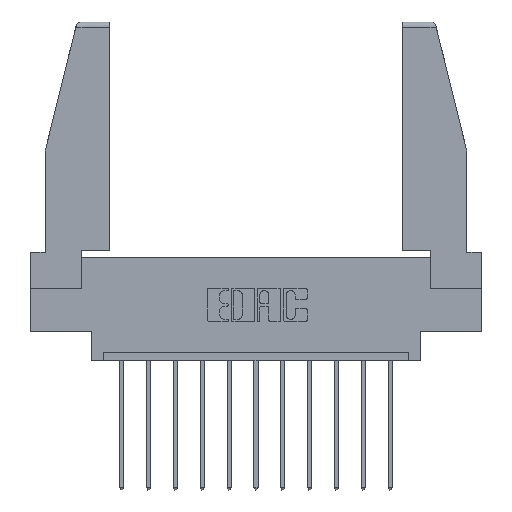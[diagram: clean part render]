
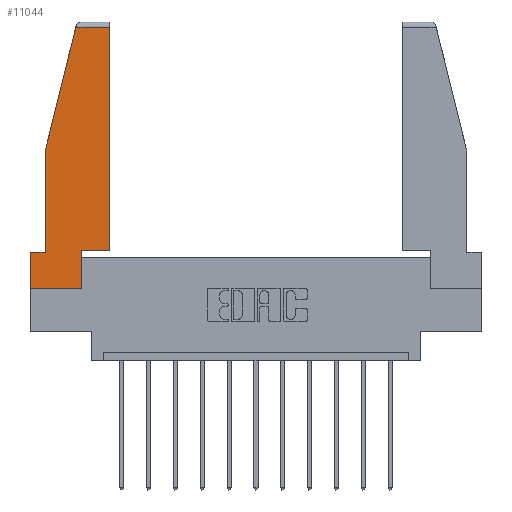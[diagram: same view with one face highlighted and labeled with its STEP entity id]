
A CAD part, top view. The second image highlights one B-rep face of the part: STEP entity #11044.
In plain terms, the highlighted planar face has unit normal (0, 0, 1).
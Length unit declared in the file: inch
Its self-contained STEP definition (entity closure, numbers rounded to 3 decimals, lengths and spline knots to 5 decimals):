
#99 = VERTEX_POINT ( 'NONE', #249 ) ;
#249 = CARTESIAN_POINT ( 'NONE',  ( 0., 0., 0. ) ) ;
#273 = VERTEX_POINT ( 'NONE', #652 ) ;
#368 = DIRECTION ( 'NONE',  ( 1., 0., 0. ) ) ;
#548 = ORIENTED_EDGE ( 'NONE', *, *, #2479, .T. ) ;
#652 = CARTESIAN_POINT ( 'NONE',  ( 0.297, 0., 0. ) ) ;
#979 = VECTOR ( 'NONE', #10877, 39.37008 ) ;
#1027 = CARTESIAN_POINT ( 'NONE',  ( 0.2636, 1.52, 0. ) ) ;
#1032 = PLANE ( 'NONE',  #13003 ) ;
#1252 = VERTEX_POINT ( 'NONE', #6017 ) ;
#1619 = VERTEX_POINT ( 'NONE', #10831 ) ;
#1668 = VERTEX_POINT ( 'NONE', #13361 ) ;
#1780 = EDGE_CURVE ( 'NONE', #8376, #1252, #3135, .T. ) ;
#1925 = VERTEX_POINT ( 'NONE', #1027 ) ;
#1956 = CARTESIAN_POINT ( 'NONE',  ( 0.086, 0.21, 0. ) ) ;
#2058 = EDGE_LOOP ( 'NONE', ( #2463, #4514, #11851, #9837, #10548, #11877, #548, #4662, #4446 ) ) ;
#2217 = CARTESIAN_POINT ( 'NONE',  ( 0., 0., 0. ) ) ;
#2333 = LINE ( 'NONE', #14441, #11269 ) ;
#2463 = ORIENTED_EDGE ( 'NONE', *, *, #7764, .T. ) ;
#2479 = EDGE_CURVE ( 'NONE', #99, #273, #2921, .T. ) ;
#2921 = LINE ( 'NONE', #9911, #979 ) ;
#3043 = DIRECTION ( 'NONE',  ( -1., 0., 0. ) ) ;
#3135 = LINE ( 'NONE', #3765, #7431 ) ;
#3298 = CARTESIAN_POINT ( 'NONE',  ( 0.461, 0.223, 0. ) ) ;
#3741 = VERTEX_POINT ( 'NONE', #9821 ) ;
#3765 = CARTESIAN_POINT ( 'NONE',  ( 0., 0.21, 0. ) ) ;
#3858 = CARTESIAN_POINT ( 'NONE',  ( 0.297, 0.223, 0. ) ) ;
#3889 = DIRECTION ( 'NONE',  ( 0., 1., 0. ) ) ;
#4357 = VECTOR ( 'NONE', #8393, 39.37008 ) ;
#4446 = ORIENTED_EDGE ( 'NONE', *, *, #6600, .T. ) ;
#4514 = ORIENTED_EDGE ( 'NONE', *, *, #7232, .T. ) ;
#4662 = ORIENTED_EDGE ( 'NONE', *, *, #6909, .T. ) ;
#4906 = LINE ( 'NONE', #8786, #7953 ) ;
#5249 = DIRECTION ( 'NONE',  ( 0., -1., 0. ) ) ;
#5335 = LINE ( 'NONE', #14324, #12324 ) ;
#5542 = LINE ( 'NONE', #8538, #11627 ) ;
#5747 = LINE ( 'NONE', #3858, #14504 ) ;
#6017 = CARTESIAN_POINT ( 'NONE',  ( 0., 0.21, 0. ) ) ;
#6600 = EDGE_CURVE ( 'NONE', #3741, #9250, #5747, .T. ) ;
#6627 = DIRECTION ( 'NONE',  ( 1., 0., 0. ) ) ;
#6716 = FACE_OUTER_BOUND ( 'NONE', #2058, .T. ) ;
#6909 = EDGE_CURVE ( 'NONE', #273, #3741, #8396, .T. ) ;
#7232 = EDGE_CURVE ( 'NONE', #1668, #1925, #2333, .T. ) ;
#7318 = DIRECTION ( 'NONE',  ( -1., 0., 0. ) ) ;
#7431 = VECTOR ( 'NONE', #7318, 39.37008 ) ;
#7764 = EDGE_CURVE ( 'NONE', #9250, #1668, #5335, .T. ) ;
#7953 = VECTOR ( 'NONE', #5249, 39.37008 ) ;
#8376 = VERTEX_POINT ( 'NONE', #1956 ) ;
#8393 = DIRECTION ( 'NONE',  ( 0., -1., 0. ) ) ;
#8396 = LINE ( 'NONE', #10964, #13790 ) ;
#8538 = CARTESIAN_POINT ( 'NONE',  ( 0.271, 1.55, 0. ) ) ;
#8786 = CARTESIAN_POINT ( 'NONE',  ( 0.086, 0.8, 0. ) ) ;
#8989 = DIRECTION ( 'NONE',  ( 0., 0., 1. ) ) ;
#9250 = VERTEX_POINT ( 'NONE', #3298 ) ;
#9790 = DIRECTION ( 'NONE',  ( -0.239, -0.971, 0. ) ) ;
#9821 = CARTESIAN_POINT ( 'NONE',  ( 0.297, 0.223, 0. ) ) ;
#9837 = ORIENTED_EDGE ( 'NONE', *, *, #10958, .T. ) ;
#9911 = CARTESIAN_POINT ( 'NONE',  ( 0., 0., 0. ) ) ;
#10000 = DIRECTION ( 'NONE',  ( 0., 1., 0. ) ) ;
#10077 = LINE ( 'NONE', #10902, #4357 ) ;
#10211 = EDGE_CURVE ( 'NONE', #1252, #99, #10077, .T. ) ;
#10548 = ORIENTED_EDGE ( 'NONE', *, *, #1780, .T. ) ;
#10831 = CARTESIAN_POINT ( 'NONE',  ( 0.086, 0.8, 0. ) ) ;
#10877 = DIRECTION ( 'NONE',  ( 1., 0., 0. ) ) ;
#10902 = CARTESIAN_POINT ( 'NONE',  ( 0., 0.21, 0. ) ) ;
#10958 = EDGE_CURVE ( 'NONE', #1619, #8376, #4906, .T. ) ;
#10964 = CARTESIAN_POINT ( 'NONE',  ( 0.297, 0., 0. ) ) ;
#11044 = ADVANCED_FACE ( 'NONE', ( #6716 ), #1032, .T. ) ;
#11269 = VECTOR ( 'NONE', #3043, 39.37008 ) ;
#11627 = VECTOR ( 'NONE', #9790, 39.37008 ) ;
#11851 = ORIENTED_EDGE ( 'NONE', *, *, #14744, .T. ) ;
#11877 = ORIENTED_EDGE ( 'NONE', *, *, #10211, .T. ) ;
#12324 = VECTOR ( 'NONE', #3889, 39.37008 ) ;
#13003 = AXIS2_PLACEMENT_3D ( 'NONE', #2217, #8989, #6627 ) ;
#13361 = CARTESIAN_POINT ( 'NONE',  ( 0.461, 1.52, 0. ) ) ;
#13790 = VECTOR ( 'NONE', #10000, 39.37008 ) ;
#14324 = CARTESIAN_POINT ( 'NONE',  ( 0.461, 0.223, 0. ) ) ;
#14441 = CARTESIAN_POINT ( 'NONE',  ( 0., 1.52, 0. ) ) ;
#14504 = VECTOR ( 'NONE', #368, 39.37008 ) ;
#14744 = EDGE_CURVE ( 'NONE', #1925, #1619, #5542, .T. ) ;
